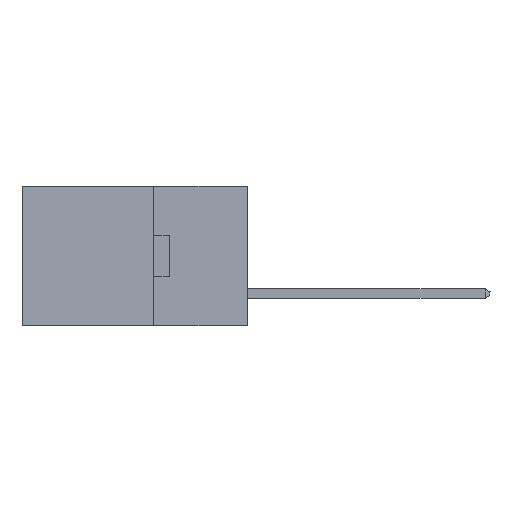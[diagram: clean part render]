
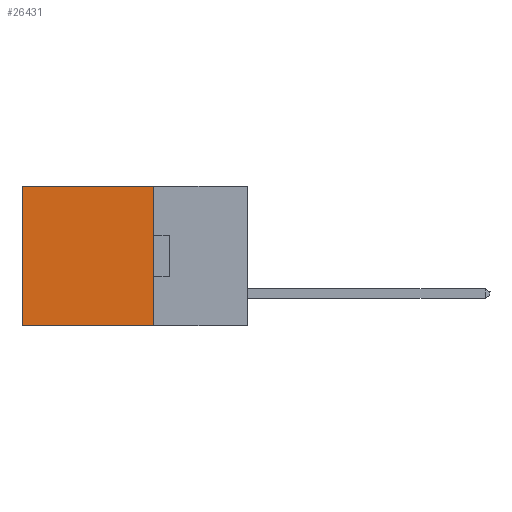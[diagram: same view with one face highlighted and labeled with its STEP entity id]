
A CAD part, left-side view. The second image highlights one B-rep face of the part: STEP entity #26431.
In plain terms, the highlighted planar face has unit normal (-1, 0, 0).
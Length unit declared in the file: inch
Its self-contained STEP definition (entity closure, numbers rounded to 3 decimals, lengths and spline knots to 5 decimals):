
#1461 = DIRECTION ( 'NONE',  ( 0., 0., -1. ) ) ;
#2108 = VECTOR ( 'NONE', #22104, 39.37008 ) ;
#2600 = DIRECTION ( 'NONE',  ( 0., 1., 0. ) ) ;
#2628 = EDGE_LOOP ( 'NONE', ( #17102, #22743, #4074, #12163 ) ) ;
#2931 = CARTESIAN_POINT ( 'NONE',  ( 0.2615, 0.25, -0.37 ) ) ;
#3619 = VECTOR ( 'NONE', #1461, 39.37008 ) ;
#4074 = ORIENTED_EDGE ( 'NONE', *, *, #5808, .F. ) ;
#4400 = EDGE_CURVE ( 'NONE', #11889, #12246, #17680, .T. ) ;
#4634 = CARTESIAN_POINT ( 'NONE',  ( 0.2615, 0.25, -0.37 ) ) ;
#5808 = EDGE_CURVE ( 'NONE', #23249, #16758, #21696, .T. ) ;
#5860 = VECTOR ( 'NONE', #17365, 39.37008 ) ;
#9060 = PLANE ( 'NONE',  #12157 ) ;
#11758 = LINE ( 'NONE', #13942, #2108 ) ;
#11889 = VERTEX_POINT ( 'NONE', #22263 ) ;
#12157 = AXIS2_PLACEMENT_3D ( 'NONE', #2931, #15327, #23625 ) ;
#12163 = ORIENTED_EDGE ( 'NONE', *, *, #12328, .T. ) ;
#12246 = VERTEX_POINT ( 'NONE', #15312 ) ;
#12328 = EDGE_CURVE ( 'NONE', #23249, #11889, #11758, .T. ) ;
#13555 = FACE_OUTER_BOUND ( 'NONE', #2628, .T. ) ;
#13942 = CARTESIAN_POINT ( 'NONE',  ( 0.2615, 0.25, 0. ) ) ;
#15306 = CARTESIAN_POINT ( 'NONE',  ( 0.2615, 0.25, -0.37 ) ) ;
#15312 = CARTESIAN_POINT ( 'NONE',  ( 0.2615, 0.6, -0.37 ) ) ;
#15327 = DIRECTION ( 'NONE',  ( 1., 0., 0. ) ) ;
#16758 = VERTEX_POINT ( 'NONE', #23375 ) ;
#17102 = ORIENTED_EDGE ( 'NONE', *, *, #4400, .T. ) ;
#17365 = DIRECTION ( 'NONE',  ( 0., 0., -1. ) ) ;
#17680 = LINE ( 'NONE', #25835, #3619 ) ;
#19152 = VECTOR ( 'NONE', #2600, 39.37008 ) ;
#21696 = LINE ( 'NONE', #15306, #5860 ) ;
#22104 = DIRECTION ( 'NONE',  ( 0., 1., 0. ) ) ;
#22263 = CARTESIAN_POINT ( 'NONE',  ( 0.2615, 0.6, 0. ) ) ;
#22743 = ORIENTED_EDGE ( 'NONE', *, *, #25517, .F. ) ;
#23249 = VERTEX_POINT ( 'NONE', #26111 ) ;
#23295 = LINE ( 'NONE', #4634, #19152 ) ;
#23375 = CARTESIAN_POINT ( 'NONE',  ( 0.2615, 0.25, -0.37 ) ) ;
#23625 = DIRECTION ( 'NONE',  ( 0., 0., -1. ) ) ;
#25517 = EDGE_CURVE ( 'NONE', #16758, #12246, #23295, .T. ) ;
#25835 = CARTESIAN_POINT ( 'NONE',  ( 0.2615, 0.6, -0.37 ) ) ;
#26111 = CARTESIAN_POINT ( 'NONE',  ( 0.2615, 0.25, 0. ) ) ;
#26431 = ADVANCED_FACE ( 'NONE', ( #13555 ), #9060, .F. ) ;
